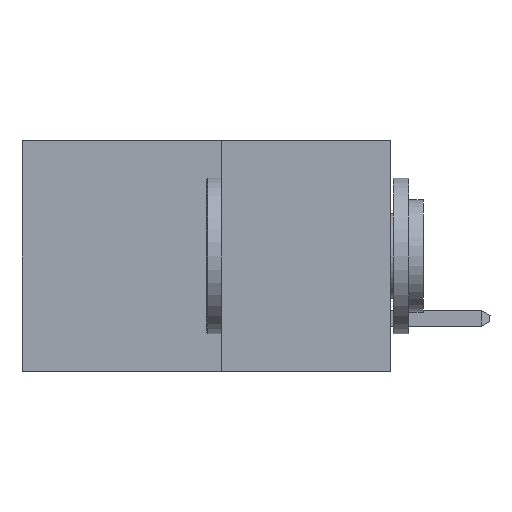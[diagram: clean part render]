
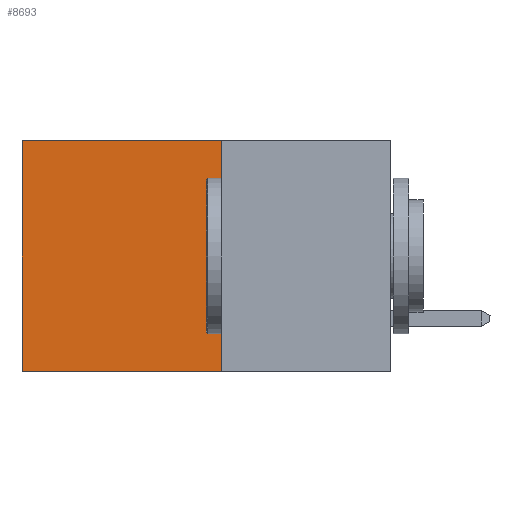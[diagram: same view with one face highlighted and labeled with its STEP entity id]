
A CAD part, left-side view. The second image highlights one B-rep face of the part: STEP entity #8693.
In plain terms, the highlighted planar face has unit normal (-1, 0, 0).
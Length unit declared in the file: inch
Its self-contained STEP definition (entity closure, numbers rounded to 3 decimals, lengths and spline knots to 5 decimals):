
#580 = CARTESIAN_POINT ( 'NONE',  ( 0.277, 0.59, 0. ) ) ;
#1102 = VECTOR ( 'NONE', #7237, 39.37008 ) ;
#1147 = AXIS2_PLACEMENT_3D ( 'NONE', #4394, #2175, #7425 ) ;
#1213 = EDGE_LOOP ( 'NONE', ( #8417, #4032, #5411, #2859 ) ) ;
#1288 = VERTEX_POINT ( 'NONE', #3160 ) ;
#1295 = VECTOR ( 'NONE', #5020, 39.37008 ) ;
#1907 = VERTEX_POINT ( 'NONE', #580 ) ;
#2120 = EDGE_CURVE ( 'NONE', #1288, #5898, #5066, .T. ) ;
#2175 = DIRECTION ( 'NONE',  ( 1., 0., 0. ) ) ;
#2859 = ORIENTED_EDGE ( 'NONE', *, *, #3119, .T. ) ;
#3083 = VERTEX_POINT ( 'NONE', #4873 ) ;
#3119 = EDGE_CURVE ( 'NONE', #1288, #1907, #8204, .T. ) ;
#3160 = CARTESIAN_POINT ( 'NONE',  ( 0.277, 0.27, 0. ) ) ;
#3269 = VECTOR ( 'NONE', #9647, 39.37008 ) ;
#4032 = ORIENTED_EDGE ( 'NONE', *, *, #6438, .F. ) ;
#4394 = CARTESIAN_POINT ( 'NONE',  ( 0.277, 0.27, -0.37 ) ) ;
#4414 = CARTESIAN_POINT ( 'NONE',  ( 0.277, 0.27, -0.37 ) ) ;
#4656 = VECTOR ( 'NONE', #9034, 39.37008 ) ;
#4873 = CARTESIAN_POINT ( 'NONE',  ( 0.277, 0.59, -0.37 ) ) ;
#4901 = CARTESIAN_POINT ( 'NONE',  ( 0.277, 0.27, -0.37 ) ) ;
#5017 = LINE ( 'NONE', #4414, #3269 ) ;
#5020 = DIRECTION ( 'NONE',  ( 0., 0., -1. ) ) ;
#5066 = LINE ( 'NONE', #4901, #1102 ) ;
#5138 = CARTESIAN_POINT ( 'NONE',  ( 0.277, 0.27, 0. ) ) ;
#5411 = ORIENTED_EDGE ( 'NONE', *, *, #2120, .F. ) ;
#5898 = VERTEX_POINT ( 'NONE', #6043 ) ;
#6043 = CARTESIAN_POINT ( 'NONE',  ( 0.277, 0.27, -0.37 ) ) ;
#6438 = EDGE_CURVE ( 'NONE', #5898, #3083, #5017, .T. ) ;
#6686 = PLANE ( 'NONE',  #1147 ) ;
#6919 = EDGE_CURVE ( 'NONE', #1907, #3083, #8784, .T. ) ;
#7237 = DIRECTION ( 'NONE',  ( 0., 0., -1. ) ) ;
#7425 = DIRECTION ( 'NONE',  ( 0., 0., -1. ) ) ;
#8034 = CARTESIAN_POINT ( 'NONE',  ( 0.277, 0.59, -0.37 ) ) ;
#8204 = LINE ( 'NONE', #5138, #4656 ) ;
#8417 = ORIENTED_EDGE ( 'NONE', *, *, #6919, .T. ) ;
#8693 = ADVANCED_FACE ( 'NONE', ( #9049 ), #6686, .F. ) ;
#8784 = LINE ( 'NONE', #8034, #1295 ) ;
#9034 = DIRECTION ( 'NONE',  ( 0., 1., 0. ) ) ;
#9049 = FACE_OUTER_BOUND ( 'NONE', #1213, .T. ) ;
#9647 = DIRECTION ( 'NONE',  ( 0., 1., 0. ) ) ;
